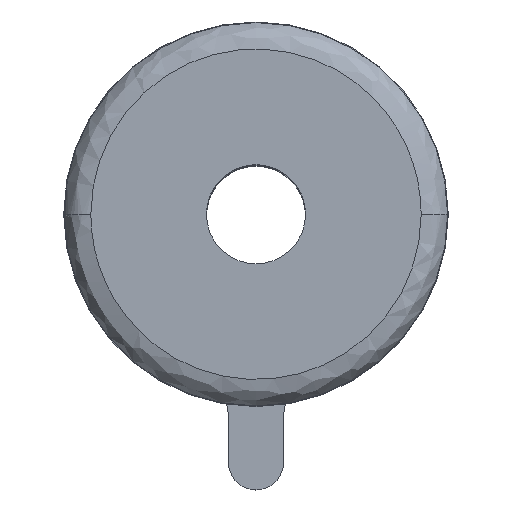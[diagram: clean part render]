
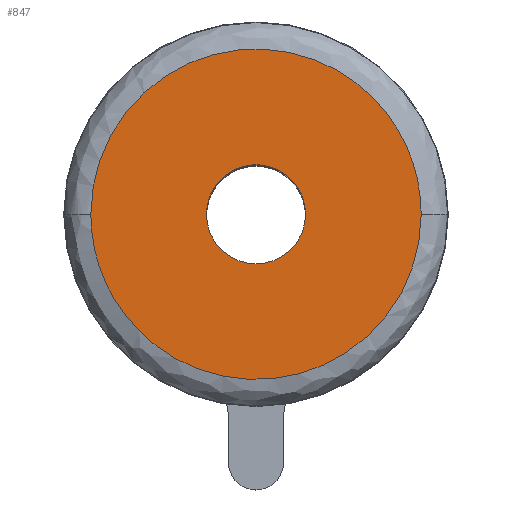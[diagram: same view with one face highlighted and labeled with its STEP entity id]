
A CAD part, top view. The second image highlights one B-rep face of the part: STEP entity #847.
In plain terms, the highlighted planar face has unit normal (0, 0, 1).
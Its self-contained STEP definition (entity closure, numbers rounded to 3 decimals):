
#847 = ADVANCED_FACE ( 'NONE', ( #1494, #1490 ), #2524, .T. ) ;
#900 = EDGE_CURVE ( 'NONE', #3818, #3784, #1119, .T. ) ;
#948 = EDGE_CURVE ( 'NONE', #3701, #3702, #3542, .T. ) ;
#967 = EDGE_CURVE ( 'NONE', #3702, #3701, #3546, .T. ) ;
#969 = EDGE_CURVE ( 'NONE', #3784, #3818, #1151, .T. ) ;
#1119 = CIRCLE ( 'NONE', #1539, 4.572 ) ;
#1151 = CIRCLE ( 'NONE', #1615, 4.572 ) ;
#1490 = FACE_BOUND ( 'NONE', #3646, .T. ) ;
#1494 = FACE_OUTER_BOUND ( 'NONE', #3648, .T. ) ;
#1509 = AXIS2_PLACEMENT_3D ( 'NONE', #2535, #2506, #2519 ) ;
#1539 = AXIS2_PLACEMENT_3D ( 'NONE', #2743, #2762, #2737 ) ;
#1615 = AXIS2_PLACEMENT_3D ( 'NONE', #3121, #3122, #3123 ) ;
#2094 = CARTESIAN_POINT ( 'NONE',  ( -15.24, 0., 63.5 ) ) ;
#2108 = CARTESIAN_POINT ( 'NONE',  ( 15.24, 0., 63.5 ) ) ;
#2160 = CARTESIAN_POINT ( 'NONE',  ( -4.572, 0., 63.5 ) ) ;
#2186 = CARTESIAN_POINT ( 'NONE',  ( 4.572, 0., 63.5 ) ) ;
#2506 = DIRECTION ( 'NONE',  ( 0., 0., 1. ) ) ;
#2519 = DIRECTION ( 'NONE',  ( 1., 0., 0. ) ) ;
#2524 = PLANE ( 'NONE',  #1509 ) ;
#2535 = CARTESIAN_POINT ( 'NONE',  ( 0., 0., 63.5 ) ) ;
#2737 = DIRECTION ( 'NONE',  ( -1., 0., 0. ) ) ;
#2743 = CARTESIAN_POINT ( 'NONE',  ( 0., 0., 63.5 ) ) ;
#2762 = DIRECTION ( 'NONE',  ( 0., 0., -1. ) ) ;
#2959 = CARTESIAN_POINT ( 'NONE',  ( 15.24, -30.48, 63.5 ) ) ;
#2962 = CARTESIAN_POINT ( 'NONE',  ( -15.24, 0., 63.5 ) ) ;
#2964 = CARTESIAN_POINT ( 'NONE',  ( 15.24, 0., 63.5 ) ) ;
#2969 = CARTESIAN_POINT ( 'NONE',  ( -15.24, -30.48, 63.5 ) ) ;
#3083 = CARTESIAN_POINT ( 'NONE',  ( -15.24, 0., 63.5 ) ) ;
#3113 = CARTESIAN_POINT ( 'NONE',  ( 15.24, 0., 63.5 ) ) ;
#3120 = CARTESIAN_POINT ( 'NONE',  ( 15.24, 30.48, 63.5 ) ) ;
#3121 = CARTESIAN_POINT ( 'NONE',  ( 0., 0., 63.5 ) ) ;
#3122 = DIRECTION ( 'NONE',  ( 0., 0., -1. ) ) ;
#3123 = DIRECTION ( 'NONE',  ( -1., 0., 0. ) ) ;
#3128 = CARTESIAN_POINT ( 'NONE',  ( -15.24, 30.48, 63.5 ) ) ;
#3542 =( BOUNDED_CURVE ( )  B_SPLINE_CURVE ( 3, ( #2964, #2959, #2969, #2962 ),
 .UNSPECIFIED., .F., .F. ) 
 B_SPLINE_CURVE_WITH_KNOTS ( ( 4, 4 ),
 ( 0., 1. ),
 .UNSPECIFIED. ) 
 CURVE ( )  GEOMETRIC_REPRESENTATION_ITEM ( )  RATIONAL_B_SPLINE_CURVE ( ( 1., 0.333, 0.333, 1. ) ) 
 REPRESENTATION_ITEM ( '' )  );
#3546 =( BOUNDED_CURVE ( )  B_SPLINE_CURVE ( 3, ( #3083, #3128, #3120, #3113 ),
 .UNSPECIFIED., .F., .F. ) 
 B_SPLINE_CURVE_WITH_KNOTS ( ( 4, 4 ),
 ( 0., 1. ),
 .UNSPECIFIED. ) 
 CURVE ( )  GEOMETRIC_REPRESENTATION_ITEM ( )  RATIONAL_B_SPLINE_CURVE ( ( 1., 0.333, 0.333, 1. ) ) 
 REPRESENTATION_ITEM ( '' )  );
#3646 = EDGE_LOOP ( 'NONE', ( #3841, #3850 ) ) ;
#3648 = EDGE_LOOP ( 'NONE', ( #3863, #3869 ) ) ;
#3701 = VERTEX_POINT ( 'NONE', #2108 ) ;
#3702 = VERTEX_POINT ( 'NONE', #2094 ) ;
#3784 = VERTEX_POINT ( 'NONE', #2160 ) ;
#3818 = VERTEX_POINT ( 'NONE', #2186 ) ;
#3841 = ORIENTED_EDGE ( 'NONE', *, *, #969, .T. ) ;
#3850 = ORIENTED_EDGE ( 'NONE', *, *, #900, .T. ) ;
#3863 = ORIENTED_EDGE ( 'NONE', *, *, #967, .F. ) ;
#3869 = ORIENTED_EDGE ( 'NONE', *, *, #948, .F. ) ;
